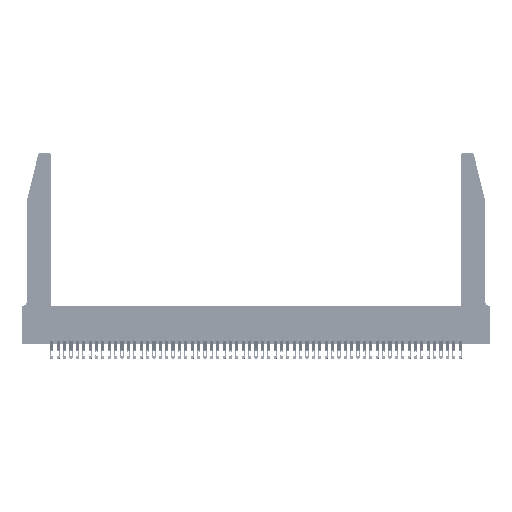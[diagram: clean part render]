
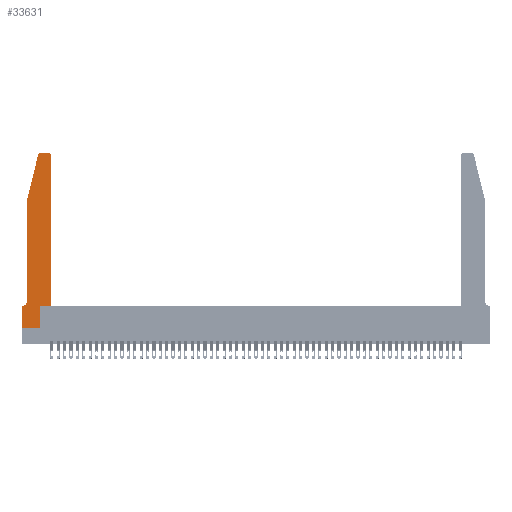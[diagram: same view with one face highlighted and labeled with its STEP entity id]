
A CAD part, top view. The second image highlights one B-rep face of the part: STEP entity #33631.
In plain terms, the highlighted planar face has unit normal (0, 0, 1).
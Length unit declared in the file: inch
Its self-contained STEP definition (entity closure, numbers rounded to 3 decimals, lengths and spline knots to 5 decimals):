
#728 = VERTEX_POINT ( 'NONE', #49245 ) ;
#1408 = CARTESIAN_POINT ( 'NONE',  ( 0., 0.35, 0.37 ) ) ;
#1804 = AXIS2_PLACEMENT_3D ( 'NONE', #10867, #51851, #47044 ) ;
#2290 = CARTESIAN_POINT ( 'NONE',  ( 0.2605, 2.75, 0.37 ) ) ;
#2918 = EDGE_CURVE ( 'NONE', #12857, #23754, #23979, .T. ) ;
#3309 = DIRECTION ( 'NONE',  ( 0., 0., 1. ) ) ;
#3827 = CARTESIAN_POINT ( 'NONE',  ( 0., 0., 0.37 ) ) ;
#5770 = CARTESIAN_POINT ( 'NONE',  ( 0.0755, 0.35, 0.37 ) ) ;
#5870 = EDGE_CURVE ( 'NONE', #49918, #6082, #14787, .T. ) ;
#6082 = VERTEX_POINT ( 'NONE', #45452 ) ;
#6306 = ORIENTED_EDGE ( 'NONE', *, *, #18977, .T. ) ;
#7244 = VECTOR ( 'NONE', #45009, 39.37008 ) ;
#8168 = LINE ( 'NONE', #9618, #36326 ) ;
#8679 = ORIENTED_EDGE ( 'NONE', *, *, #26937, .T. ) ;
#9022 = VERTEX_POINT ( 'NONE', #22656 ) ;
#9618 = CARTESIAN_POINT ( 'NONE',  ( 0.4505, 0.35, 0.37 ) ) ;
#9793 = VECTOR ( 'NONE', #21567, 39.37008 ) ;
#10217 = LINE ( 'NONE', #20594, #52483 ) ;
#10436 = ORIENTED_EDGE ( 'NONE', *, *, #19299, .T. ) ;
#10867 = CARTESIAN_POINT ( 'NONE',  ( 0.284, 2.72, 0.37 ) ) ;
#11727 = LINE ( 'NONE', #11887, #7244 ) ;
#11887 = CARTESIAN_POINT ( 'NONE',  ( 0.2865, 0.35, 0.37 ) ) ;
#12376 = DIRECTION ( 'NONE',  ( 0., -1., 0. ) ) ;
#12622 = LINE ( 'NONE', #3827, #32562 ) ;
#12857 = VERTEX_POINT ( 'NONE', #13654 ) ;
#13631 = CARTESIAN_POINT ( 'NONE',  ( 0., 0., 0.37 ) ) ;
#13650 = CARTESIAN_POINT ( 'NONE',  ( 0.0755, 0.42, 0.37 ) ) ;
#13651 = CARTESIAN_POINT ( 'NONE',  ( 0.4505, 0.35, 0.37 ) ) ;
#13654 = CARTESIAN_POINT ( 'NONE',  ( 0.284, 2.75, 0.37 ) ) ;
#13730 = DIRECTION ( 'NONE',  ( 1., 0., 0. ) ) ;
#14213 = EDGE_CURVE ( 'NONE', #728, #28248, #28930, .T. ) ;
#14390 = CARTESIAN_POINT ( 'NONE',  ( 0.0055, 0.42, 0.37 ) ) ;
#14552 = ORIENTED_EDGE ( 'NONE', *, *, #16809, .T. ) ;
#14787 = CIRCLE ( 'NONE', #15314, 0.03 ) ;
#14945 = LINE ( 'NONE', #5770, #9793 ) ;
#15314 = AXIS2_PLACEMENT_3D ( 'NONE', #31557, #3309, #15680 ) ;
#15570 = ORIENTED_EDGE ( 'NONE', *, *, #14213, .T. ) ;
#15680 = DIRECTION ( 'NONE',  ( 1., 0., 0. ) ) ;
#16809 = EDGE_CURVE ( 'NONE', #9022, #38400, #8168, .T. ) ;
#17326 = ORIENTED_EDGE ( 'NONE', *, *, #50346, .T. ) ;
#17927 = VERTEX_POINT ( 'NONE', #49973 ) ;
#18789 = AXIS2_PLACEMENT_3D ( 'NONE', #25109, #20805, #32962 ) ;
#18878 = ORIENTED_EDGE ( 'NONE', *, *, #5870, .T. ) ;
#18977 = EDGE_CURVE ( 'NONE', #17927, #9022, #11727, .T. ) ;
#19109 = EDGE_CURVE ( 'NONE', #38400, #49918, #50177, .T. ) ;
#19299 = EDGE_CURVE ( 'NONE', #46021, #32541, #14945, .T. ) ;
#20594 = CARTESIAN_POINT ( 'NONE',  ( 0.0755, 2., 0.37 ) ) ;
#20723 = VECTOR ( 'NONE', #33726, 39.37008 ) ;
#20726 = VECTOR ( 'NONE', #43778, 39.37008 ) ;
#20805 = DIRECTION ( 'NONE',  ( 0., 0., 1. ) ) ;
#21567 = DIRECTION ( 'NONE',  ( -1., 0., 0. ) ) ;
#21690 = DIRECTION ( 'NONE',  ( 1., 0., 0. ) ) ;
#21856 = CARTESIAN_POINT ( 'NONE',  ( 0., 0., 0.37 ) ) ;
#22356 = ORIENTED_EDGE ( 'NONE', *, *, #46604, .T. ) ;
#22656 = CARTESIAN_POINT ( 'NONE',  ( 0.2865, 0.35, 0.37 ) ) ;
#22737 = VERTEX_POINT ( 'NONE', #13631 ) ;
#22835 = CIRCLE ( 'NONE', #32869, 0.07 ) ;
#23754 = VERTEX_POINT ( 'NONE', #49774 ) ;
#23979 = CIRCLE ( 'NONE', #1804, 0.03 ) ;
#24393 = LINE ( 'NONE', #21856, #34008 ) ;
#25109 = CARTESIAN_POINT ( 'NONE',  ( 0., 0.35, 0.37 ) ) ;
#26582 = FACE_OUTER_BOUND ( 'NONE', #52132, .T. ) ;
#26937 = EDGE_CURVE ( 'NONE', #23754, #728, #10217, .T. ) ;
#27031 = VECTOR ( 'NONE', #45368, 39.37008 ) ;
#28248 = VERTEX_POINT ( 'NONE', #13650 ) ;
#28930 = LINE ( 'NONE', #50209, #27031 ) ;
#29559 = PLANE ( 'NONE',  #18789 ) ;
#31071 = ORIENTED_EDGE ( 'NONE', *, *, #52321, .T. ) ;
#31557 = CARTESIAN_POINT ( 'NONE',  ( 0.4205, 2.72, 0.37 ) ) ;
#32541 = VERTEX_POINT ( 'NONE', #1408 ) ;
#32562 = VECTOR ( 'NONE', #12376, 39.37008 ) ;
#32704 = ORIENTED_EDGE ( 'NONE', *, *, #2918, .T. ) ;
#32869 = AXIS2_PLACEMENT_3D ( 'NONE', #14390, #43001, #38335 ) ;
#32962 = DIRECTION ( 'NONE',  ( 1., 0., 0. ) ) ;
#33631 = ADVANCED_FACE ( 'NONE', ( #26582 ), #29559, .T. ) ;
#33726 = DIRECTION ( 'NONE',  ( 0., 1., 0. ) ) ;
#34008 = VECTOR ( 'NONE', #21690, 39.37008 ) ;
#34532 = EDGE_CURVE ( 'NONE', #6082, #12857, #41197, .T. ) ;
#36326 = VECTOR ( 'NONE', #13730, 39.37008 ) ;
#37371 = DIRECTION ( 'NONE',  ( -0.239, -0.971, 0. ) ) ;
#38054 = ORIENTED_EDGE ( 'NONE', *, *, #19109, .T. ) ;
#38335 = DIRECTION ( 'NONE',  ( -1., 0., 0. ) ) ;
#38393 = CARTESIAN_POINT ( 'NONE',  ( 0.0055, 0.35, 0.37 ) ) ;
#38400 = VERTEX_POINT ( 'NONE', #13651 ) ;
#40161 = CARTESIAN_POINT ( 'NONE',  ( 0.4505, 0.35, 0.37 ) ) ;
#41197 = LINE ( 'NONE', #2290, #20726 ) ;
#43001 = DIRECTION ( 'NONE',  ( 0., 0., -1. ) ) ;
#43041 = ORIENTED_EDGE ( 'NONE', *, *, #34532, .T. ) ;
#43778 = DIRECTION ( 'NONE',  ( -1., 0., 0. ) ) ;
#45009 = DIRECTION ( 'NONE',  ( 0., 1., 0. ) ) ;
#45368 = DIRECTION ( 'NONE',  ( 0., -1., 0. ) ) ;
#45452 = CARTESIAN_POINT ( 'NONE',  ( 0.4205, 2.75, 0.37 ) ) ;
#46021 = VERTEX_POINT ( 'NONE', #38393 ) ;
#46604 = EDGE_CURVE ( 'NONE', #28248, #46021, #22835, .T. ) ;
#47044 = DIRECTION ( 'NONE',  ( 1., 0., 0. ) ) ;
#49245 = CARTESIAN_POINT ( 'NONE',  ( 0.0755, 2., 0.37 ) ) ;
#49774 = CARTESIAN_POINT ( 'NONE',  ( 0.25487, 2.72718, 0.37 ) ) ;
#49918 = VERTEX_POINT ( 'NONE', #52323 ) ;
#49973 = CARTESIAN_POINT ( 'NONE',  ( 0.2865, 0., 0.37 ) ) ;
#50177 = LINE ( 'NONE', #40161, #20723 ) ;
#50209 = CARTESIAN_POINT ( 'NONE',  ( 0.0755, 2., 0.37 ) ) ;
#50346 = EDGE_CURVE ( 'NONE', #22737, #17927, #24393, .T. ) ;
#51851 = DIRECTION ( 'NONE',  ( 0., 0., 1. ) ) ;
#52132 = EDGE_LOOP ( 'NONE', ( #43041, #32704, #8679, #15570, #22356, #10436, #31071, #17326, #6306, #14552, #38054, #18878 ) ) ;
#52321 = EDGE_CURVE ( 'NONE', #32541, #22737, #12622, .T. ) ;
#52323 = CARTESIAN_POINT ( 'NONE',  ( 0.4505, 2.72, 0.37 ) ) ;
#52483 = VECTOR ( 'NONE', #37371, 39.37008 ) ;
